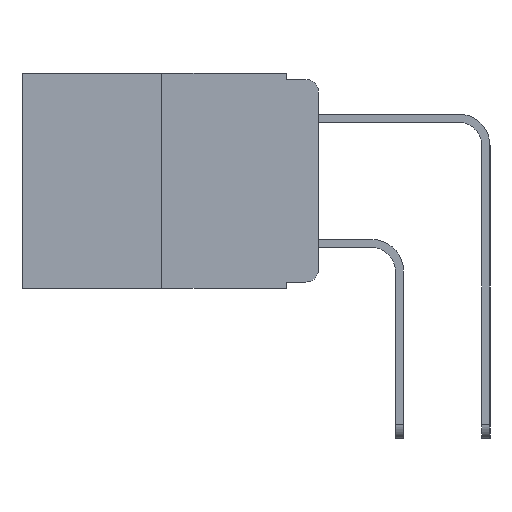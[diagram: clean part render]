
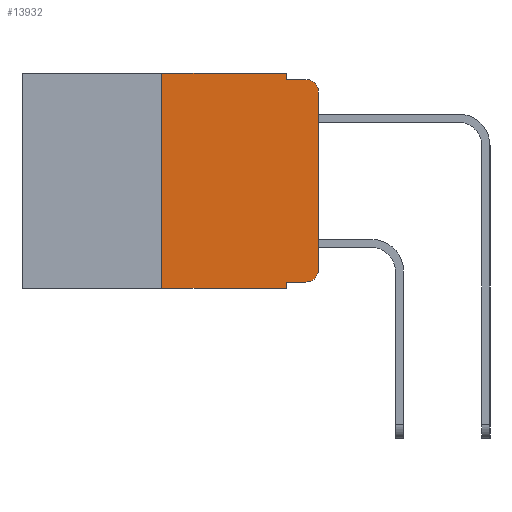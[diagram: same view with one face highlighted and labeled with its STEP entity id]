
A CAD part, left-side view. The second image highlights one B-rep face of the part: STEP entity #13932.
In plain terms, the highlighted planar face has unit normal (-1, 0, 0).
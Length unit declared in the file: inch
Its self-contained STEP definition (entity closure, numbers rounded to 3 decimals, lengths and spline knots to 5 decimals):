
#51 = DIRECTION ( 'NONE',  ( 0., -1., 0. ) ) ;
#98 = DIRECTION ( 'NONE',  ( 1., 0., 0. ) ) ;
#144 = DIRECTION ( 'NONE',  ( 0., 0., -1. ) ) ;
#235 = ORIENTED_EDGE ( 'NONE', *, *, #1853, .F. ) ;
#614 = VERTEX_POINT ( 'NONE', #10707 ) ;
#711 = VERTEX_POINT ( 'NONE', #3648 ) ;
#782 = ORIENTED_EDGE ( 'NONE', *, *, #10083, .T. ) ;
#952 = AXIS2_PLACEMENT_3D ( 'NONE', #14514, #7209, #15709 ) ;
#1596 = CARTESIAN_POINT ( 'NONE',  ( 0., 0.02, -0.333 ) ) ;
#1711 = DIRECTION ( 'NONE',  ( 0., -1., 0. ) ) ;
#1721 = ORIENTED_EDGE ( 'NONE', *, *, #8721, .F. ) ;
#1813 = LINE ( 'NONE', #11471, #11207 ) ;
#1853 = EDGE_CURVE ( 'NONE', #3398, #5342, #11099, .T. ) ;
#2238 = LINE ( 'NONE', #15479, #8418 ) ;
#2511 = VECTOR ( 'NONE', #11947, 39.37008 ) ;
#2605 = VERTEX_POINT ( 'NONE', #6870 ) ;
#2843 = EDGE_LOOP ( 'NONE', ( #4259, #6005, #235, #13081, #14594, #1721, #14947, #14567, #6154, #782 ) ) ;
#3200 = EDGE_CURVE ( 'NONE', #614, #15261, #13933, .T. ) ;
#3363 = CARTESIAN_POINT ( 'NONE',  ( 0., 0., 0. ) ) ;
#3398 = VERTEX_POINT ( 'NONE', #6074 ) ;
#3648 = CARTESIAN_POINT ( 'NONE',  ( 0., 0.25, 0. ) ) ;
#3840 = DIRECTION ( 'NONE',  ( 0., 0., -1. ) ) ;
#4259 = ORIENTED_EDGE ( 'NONE', *, *, #14940, .T. ) ;
#4960 = EDGE_CURVE ( 'NONE', #2605, #14833, #1813, .T. ) ;
#5165 = CIRCLE ( 'NONE', #6238, 0.02 ) ;
#5183 = LINE ( 'NONE', #11175, #11686 ) ;
#5282 = AXIS2_PLACEMENT_3D ( 'NONE', #7460, #98, #8681 ) ;
#5342 = VERTEX_POINT ( 'NONE', #14871 ) ;
#5601 = VECTOR ( 'NONE', #13810, 39.37008 ) ;
#5640 = FACE_OUTER_BOUND ( 'NONE', #2843, .T. ) ;
#5992 = LINE ( 'NONE', #6489, #5601 ) ;
#6005 = ORIENTED_EDGE ( 'NONE', *, *, #13289, .T. ) ;
#6031 = LINE ( 'NONE', #6163, #12142 ) ;
#6074 = CARTESIAN_POINT ( 'NONE',  ( 0., 0.051, -0.01 ) ) ;
#6154 = ORIENTED_EDGE ( 'NONE', *, *, #3200, .T. ) ;
#6163 = CARTESIAN_POINT ( 'NONE',  ( 0., 0.473, 0. ) ) ;
#6170 = CARTESIAN_POINT ( 'NONE',  ( 0., 0., -0.03 ) ) ;
#6238 = AXIS2_PLACEMENT_3D ( 'NONE', #14797, #7501, #144 ) ;
#6489 = CARTESIAN_POINT ( 'NONE',  ( 0., 0.25, 0. ) ) ;
#6784 = VERTEX_POINT ( 'NONE', #6170 ) ;
#6870 = CARTESIAN_POINT ( 'NONE',  ( 0., 0.25, -0.343 ) ) ;
#7209 = DIRECTION ( 'NONE',  ( -1., 0., 0. ) ) ;
#7460 = CARTESIAN_POINT ( 'NONE',  ( 0., 0.473, 0. ) ) ;
#7491 = VECTOR ( 'NONE', #14695, 39.37008 ) ;
#7501 = DIRECTION ( 'NONE',  ( -1., 0., 0. ) ) ;
#8418 = VECTOR ( 'NONE', #10630, 39.37008 ) ;
#8681 = DIRECTION ( 'NONE',  ( 0., 0., -1. ) ) ;
#8707 = LINE ( 'NONE', #3363, #2511 ) ;
#8721 = EDGE_CURVE ( 'NONE', #2605, #711, #5992, .T. ) ;
#9197 = CARTESIAN_POINT ( 'NONE',  ( 0., 0.051, 0. ) ) ;
#9593 = EDGE_CURVE ( 'NONE', #614, #14833, #5183, .T. ) ;
#10083 = EDGE_CURVE ( 'NONE', #15261, #10390, #5165, .T. ) ;
#10287 = VECTOR ( 'NONE', #13192, 39.37008 ) ;
#10329 = VERTEX_POINT ( 'NONE', #9197 ) ;
#10347 = CARTESIAN_POINT ( 'NONE',  ( 0., 0.051, -0.343 ) ) ;
#10390 = VERTEX_POINT ( 'NONE', #12948 ) ;
#10451 = EDGE_CURVE ( 'NONE', #10329, #3398, #2238, .T. ) ;
#10630 = DIRECTION ( 'NONE',  ( 0., 0., -1. ) ) ;
#10707 = CARTESIAN_POINT ( 'NONE',  ( 0., 0.051, -0.333 ) ) ;
#11099 = LINE ( 'NONE', #13488, #7491 ) ;
#11175 = CARTESIAN_POINT ( 'NONE',  ( 0., 0.051, 0. ) ) ;
#11207 = VECTOR ( 'NONE', #1711, 39.37008 ) ;
#11471 = CARTESIAN_POINT ( 'NONE',  ( 0., 0.473, -0.343 ) ) ;
#11686 = VECTOR ( 'NONE', #3840, 39.37008 ) ;
#11947 = DIRECTION ( 'NONE',  ( 0., 0., 1. ) ) ;
#12142 = VECTOR ( 'NONE', #51, 39.37008 ) ;
#12360 = CIRCLE ( 'NONE', #952, 0.02 ) ;
#12655 = CARTESIAN_POINT ( 'NONE',  ( 0., 0.051, -0.333 ) ) ;
#12948 = CARTESIAN_POINT ( 'NONE',  ( 0., 0., -0.313 ) ) ;
#13081 = ORIENTED_EDGE ( 'NONE', *, *, #10451, .F. ) ;
#13192 = DIRECTION ( 'NONE',  ( 0., -1., 0. ) ) ;
#13289 = EDGE_CURVE ( 'NONE', #6784, #5342, #12360, .T. ) ;
#13488 = CARTESIAN_POINT ( 'NONE',  ( 0., 0.051, -0.01 ) ) ;
#13810 = DIRECTION ( 'NONE',  ( 0., 0., 1. ) ) ;
#13891 = EDGE_CURVE ( 'NONE', #711, #10329, #6031, .T. ) ;
#13932 = ADVANCED_FACE ( 'NONE', ( #5640 ), #14749, .F. ) ;
#13933 = LINE ( 'NONE', #12655, #10287 ) ;
#14514 = CARTESIAN_POINT ( 'NONE',  ( 0., 0.02, -0.03 ) ) ;
#14567 = ORIENTED_EDGE ( 'NONE', *, *, #9593, .F. ) ;
#14594 = ORIENTED_EDGE ( 'NONE', *, *, #13891, .F. ) ;
#14695 = DIRECTION ( 'NONE',  ( 0., -1., 0. ) ) ;
#14749 = PLANE ( 'NONE',  #5282 ) ;
#14797 = CARTESIAN_POINT ( 'NONE',  ( 0., 0.02, -0.313 ) ) ;
#14833 = VERTEX_POINT ( 'NONE', #10347 ) ;
#14871 = CARTESIAN_POINT ( 'NONE',  ( 0., 0.02, -0.01 ) ) ;
#14940 = EDGE_CURVE ( 'NONE', #10390, #6784, #8707, .T. ) ;
#14947 = ORIENTED_EDGE ( 'NONE', *, *, #4960, .T. ) ;
#15261 = VERTEX_POINT ( 'NONE', #1596 ) ;
#15479 = CARTESIAN_POINT ( 'NONE',  ( 0., 0.051, 0. ) ) ;
#15709 = DIRECTION ( 'NONE',  ( 0., 0., -1. ) ) ;
